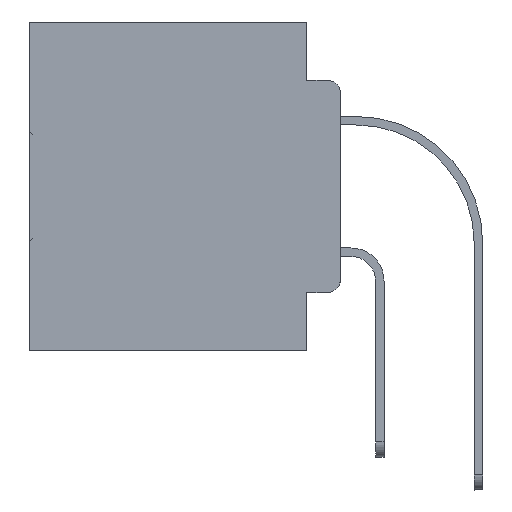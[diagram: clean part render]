
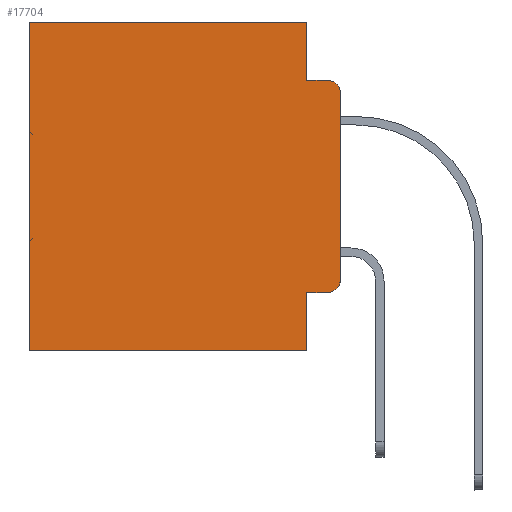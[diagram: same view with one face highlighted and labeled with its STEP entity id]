
A CAD part, left-side view. The second image highlights one B-rep face of the part: STEP entity #17704.
In plain terms, the highlighted planar face has unit normal (-1, 0, 0).
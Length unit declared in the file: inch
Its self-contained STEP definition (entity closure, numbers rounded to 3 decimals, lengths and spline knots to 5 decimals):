
#532 = FACE_OUTER_BOUND ( 'NONE', #28096, .T. ) ;
#564 = CARTESIAN_POINT ( 'NONE',  ( 0.298, 0.051, -0.5 ) ) ;
#879 = PLANE ( 'NONE',  #2002 ) ;
#1260 = VECTOR ( 'NONE', #34079, 39.37008 ) ;
#1448 = CARTESIAN_POINT ( 'NONE',  ( 0.298, 0.051, -0.0885 ) ) ;
#1501 = VERTEX_POINT ( 'NONE', #24419 ) ;
#2002 = AXIS2_PLACEMENT_3D ( 'NONE', #8617, #11495, #11846 ) ;
#2413 = LINE ( 'NONE', #35092, #17196 ) ;
#3250 = EDGE_CURVE ( 'NONE', #1501, #8611, #11947, .T. ) ;
#4475 = AXIS2_PLACEMENT_3D ( 'NONE', #27755, #33145, #8534 ) ;
#4489 = CARTESIAN_POINT ( 'NONE',  ( 0.298, 0., 0. ) ) ;
#4607 = ORIENTED_EDGE ( 'NONE', *, *, #13370, .T. ) ;
#4612 = LINE ( 'NONE', #15730, #13445 ) ;
#4637 = ORIENTED_EDGE ( 'NONE', *, *, #33627, .F. ) ;
#4944 = CARTESIAN_POINT ( 'NONE',  ( 0.298, 0.051, 0. ) ) ;
#5000 = DIRECTION ( 'NONE',  ( 0., 1., 0. ) ) ;
#5300 = ORIENTED_EDGE ( 'NONE', *, *, #34698, .T. ) ;
#5409 = DIRECTION ( 'NONE',  ( 0., 0., -1. ) ) ;
#5431 = VECTOR ( 'NONE', #12949, 39.37008 ) ;
#6792 = CARTESIAN_POINT ( 'NONE',  ( 0.298, 0.051, -0.0885 ) ) ;
#6839 = LINE ( 'NONE', #1448, #5431 ) ;
#6892 = VECTOR ( 'NONE', #5409, 39.37008 ) ;
#7309 = VERTEX_POINT ( 'NONE', #33792 ) ;
#7357 = LINE ( 'NONE', #4489, #19531 ) ;
#8047 = CARTESIAN_POINT ( 'NONE',  ( 0.298, 0., -0.5 ) ) ;
#8534 = DIRECTION ( 'NONE',  ( 0., 0., -1. ) ) ;
#8611 = VERTEX_POINT ( 'NONE', #30945 ) ;
#8617 = CARTESIAN_POINT ( 'NONE',  ( 0.298, 0., 0. ) ) ;
#8864 = VERTEX_POINT ( 'NONE', #18697 ) ;
#10389 = EDGE_CURVE ( 'NONE', #12919, #34107, #13626, .T. ) ;
#11019 = EDGE_CURVE ( 'NONE', #15561, #34107, #2413, .T. ) ;
#11495 = DIRECTION ( 'NONE',  ( 1., 0., 0. ) ) ;
#11727 = VERTEX_POINT ( 'NONE', #31447 ) ;
#11834 = CARTESIAN_POINT ( 'NONE',  ( 0.298, 0., 0. ) ) ;
#11841 = EDGE_CURVE ( 'NONE', #1501, #7309, #7357, .T. ) ;
#11846 = DIRECTION ( 'NONE',  ( 0., 0., -1. ) ) ;
#11947 = CIRCLE ( 'NONE', #4475, 0.02 ) ;
#12919 = VERTEX_POINT ( 'NONE', #564 ) ;
#12949 = DIRECTION ( 'NONE',  ( 0., -1., 0. ) ) ;
#13059 = DIRECTION ( 'NONE',  ( 0., 0., -1. ) ) ;
#13146 = ORIENTED_EDGE ( 'NONE', *, *, #10389, .F. ) ;
#13370 = EDGE_CURVE ( 'NONE', #32930, #15561, #28535, .T. ) ;
#13445 = VECTOR ( 'NONE', #13059, 39.37008 ) ;
#13626 = LINE ( 'NONE', #8047, #29765 ) ;
#13687 = EDGE_CURVE ( 'NONE', #11727, #7309, #21958, .T. ) ;
#13696 = LINE ( 'NONE', #30219, #6892 ) ;
#15561 = VERTEX_POINT ( 'NONE', #34179 ) ;
#15730 = CARTESIAN_POINT ( 'NONE',  ( 0.298, 0.051, 0. ) ) ;
#16044 = ORIENTED_EDGE ( 'NONE', *, *, #13687, .T. ) ;
#17196 = VECTOR ( 'NONE', #21443, 39.37008 ) ;
#17337 = EDGE_CURVE ( 'NONE', #17798, #8611, #6839, .T. ) ;
#17704 = ADVANCED_FACE ( 'NONE', ( #532 ), #879, .F. ) ;
#17798 = VERTEX_POINT ( 'NONE', #6792 ) ;
#18323 = DIRECTION ( 'NONE',  ( 0., 0., -1. ) ) ;
#18524 = ORIENTED_EDGE ( 'NONE', *, *, #20588, .F. ) ;
#18697 = CARTESIAN_POINT ( 'NONE',  ( 0.298, 0.051, -0.4115 ) ) ;
#19531 = VECTOR ( 'NONE', #18323, 39.37008 ) ;
#20588 = EDGE_CURVE ( 'NONE', #32930, #17798, #4612, .T. ) ;
#21443 = DIRECTION ( 'NONE',  ( 0., 0., -1. ) ) ;
#21958 = CIRCLE ( 'NONE', #27693, 0.02 ) ;
#23109 = ORIENTED_EDGE ( 'NONE', *, *, #3250, .T. ) ;
#24419 = CARTESIAN_POINT ( 'NONE',  ( 0.298, 0., -0.1085 ) ) ;
#25043 = ORIENTED_EDGE ( 'NONE', *, *, #11019, .T. ) ;
#25841 = CARTESIAN_POINT ( 'NONE',  ( 0.298, 0.473, -0.5 ) ) ;
#26642 = CARTESIAN_POINT ( 'NONE',  ( 0.298, 0.051, -0.4115 ) ) ;
#27000 = DIRECTION ( 'NONE',  ( 0., -1., 0. ) ) ;
#27224 = DIRECTION ( 'NONE',  ( -1., 0., 0. ) ) ;
#27245 = CARTESIAN_POINT ( 'NONE',  ( 0.298, 0.02, -0.3915 ) ) ;
#27693 = AXIS2_PLACEMENT_3D ( 'NONE', #27245, #27224, #27790 ) ;
#27755 = CARTESIAN_POINT ( 'NONE',  ( 0.298, 0.02, -0.1085 ) ) ;
#27790 = DIRECTION ( 'NONE',  ( 0., 0., -1. ) ) ;
#28096 = EDGE_LOOP ( 'NONE', ( #31971, #23109, #28261, #18524, #4607, #25043, #13146, #4637, #5300, #16044 ) ) ;
#28261 = ORIENTED_EDGE ( 'NONE', *, *, #17337, .F. ) ;
#28535 = LINE ( 'NONE', #11834, #1260 ) ;
#29347 = LINE ( 'NONE', #26642, #35042 ) ;
#29765 = VECTOR ( 'NONE', #5000, 39.37008 ) ;
#30219 = CARTESIAN_POINT ( 'NONE',  ( 0.298, 0.051, 0. ) ) ;
#30945 = CARTESIAN_POINT ( 'NONE',  ( 0.298, 0.02, -0.0885 ) ) ;
#31447 = CARTESIAN_POINT ( 'NONE',  ( 0.298, 0.02, -0.4115 ) ) ;
#31971 = ORIENTED_EDGE ( 'NONE', *, *, #11841, .F. ) ;
#32930 = VERTEX_POINT ( 'NONE', #4944 ) ;
#33145 = DIRECTION ( 'NONE',  ( -1., 0., 0. ) ) ;
#33627 = EDGE_CURVE ( 'NONE', #8864, #12919, #13696, .T. ) ;
#33792 = CARTESIAN_POINT ( 'NONE',  ( 0.298, 0., -0.3915 ) ) ;
#34079 = DIRECTION ( 'NONE',  ( 0., 1., 0. ) ) ;
#34107 = VERTEX_POINT ( 'NONE', #25841 ) ;
#34179 = CARTESIAN_POINT ( 'NONE',  ( 0.298, 0.473, 0. ) ) ;
#34698 = EDGE_CURVE ( 'NONE', #8864, #11727, #29347, .T. ) ;
#35042 = VECTOR ( 'NONE', #27000, 39.37008 ) ;
#35092 = CARTESIAN_POINT ( 'NONE',  ( 0.298, 0.473, 0. ) ) ;
